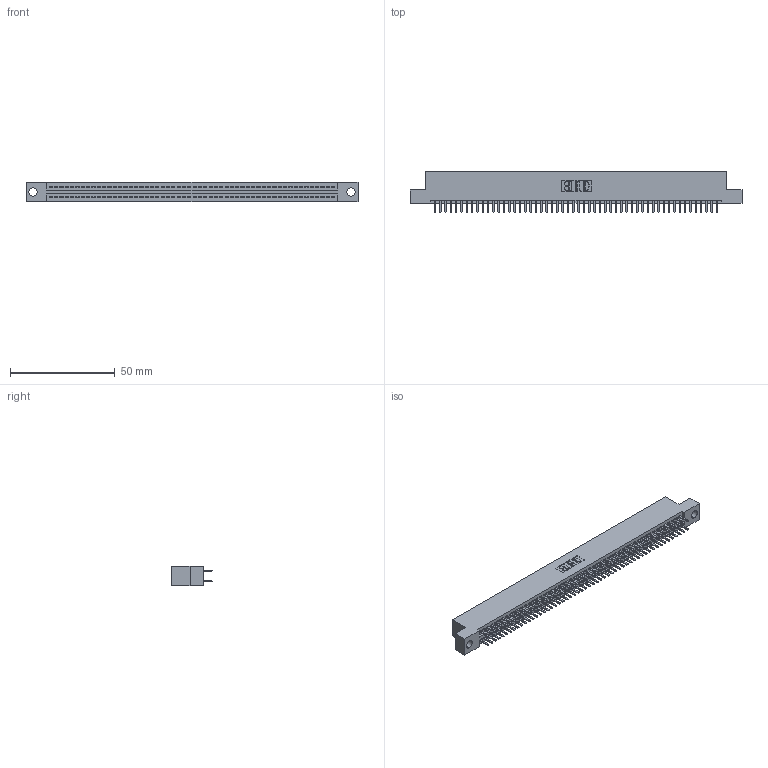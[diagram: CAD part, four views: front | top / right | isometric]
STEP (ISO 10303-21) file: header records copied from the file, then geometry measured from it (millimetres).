
FILE_DESCRIPTION (( 'STEP AP203' ), '1' );
FILE_NAME ('345-108-520-204.STEP', '2021-05-21T14:24:23', ( '' ), ( '' ), 'SwSTEP 2.0', 'SolidWorks 2020', '' );
FILE_SCHEMA (( 'CONFIG_CONTROL_DESIGN' ));
Length unit declared in the file: inch
Products named in the file (3): 345 Part_Flush Mounting Lugs - 0.156 Dia-TI; 345-292-001_345-293-120; 345-108-520-204
Assembly tree (109 placements, depth 2):
  345-108-520-204
    345 Part_Flush Mounting Lugs - 0.156 Dia-TI
    345-292-001_345-293-120  x108
Bounding box: 158.37 x 19.68 x 9.4 mm (x, y, z)
Volume: 15342.1 mm3; surface area: 22661.2 mm2
Topology: 109 solids, 109 shells, 5972 faces, 17333 edges, 11266 vertices
Faces by surface type: plane 3874, cylinder 2098
Entity records: 41287 total; most frequent: CARTESIAN_POINT 6926, ORIENTED_EDGE 6846, DIRECTION 6079, EDGE_CURVE 3423, VECTOR 3071, LINE 3071, VERTEX_POINT 2278, AXIS2_PLACEMENT_3D 1504
